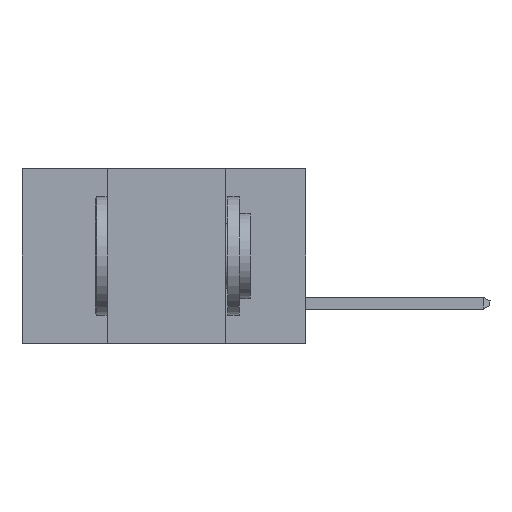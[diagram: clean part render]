
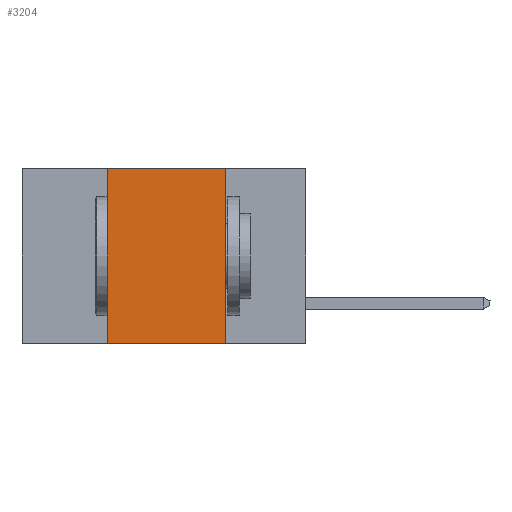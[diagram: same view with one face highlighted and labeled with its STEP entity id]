
A CAD part, left-side view. The second image highlights one B-rep face of the part: STEP entity #3204.
In plain terms, the highlighted planar face has unit normal (-1, 0, 0).
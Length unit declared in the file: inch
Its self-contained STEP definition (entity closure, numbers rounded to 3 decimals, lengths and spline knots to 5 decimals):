
#108 = VECTOR ( 'NONE', #5149, 39.37008 ) ;
#571 = CARTESIAN_POINT ( 'NONE',  ( 0., 0.42, 0. ) ) ;
#929 = LINE ( 'NONE', #991, #108 ) ;
#991 = CARTESIAN_POINT ( 'NONE',  ( 0., 0.6, 0. ) ) ;
#1037 = EDGE_CURVE ( 'NONE', #2066, #2470, #2763, .T. ) ;
#1097 = FACE_OUTER_BOUND ( 'NONE', #8620, .T. ) ;
#1545 = DIRECTION ( 'NONE',  ( 0., 0., -1. ) ) ;
#2066 = VERTEX_POINT ( 'NONE', #9506 ) ;
#2470 = VERTEX_POINT ( 'NONE', #571 ) ;
#2763 = LINE ( 'NONE', #6127, #11078 ) ;
#3100 = EDGE_CURVE ( 'NONE', #2066, #4912, #9475, .T. ) ;
#3168 = ORIENTED_EDGE ( 'NONE', *, *, #1037, .F. ) ;
#3204 = ADVANCED_FACE ( 'NONE', ( #1097 ), #3468, .F. ) ;
#3291 = CARTESIAN_POINT ( 'NONE',  ( 0., 0.17, -0.37 ) ) ;
#3309 = CARTESIAN_POINT ( 'NONE',  ( 0., 0.6, 0. ) ) ;
#3468 = PLANE ( 'NONE',  #12952 ) ;
#3511 = CARTESIAN_POINT ( 'NONE',  ( 0., 0.17, 0. ) ) ;
#4259 = DIRECTION ( 'NONE',  ( 0., -1., 0. ) ) ;
#4912 = VERTEX_POINT ( 'NONE', #3291 ) ;
#5149 = DIRECTION ( 'NONE',  ( 0., -1., 0. ) ) ;
#6127 = CARTESIAN_POINT ( 'NONE',  ( 0., 0.42, -0.37 ) ) ;
#6319 = CARTESIAN_POINT ( 'NONE',  ( 0., 0.6, -0.37 ) ) ;
#6654 = DIRECTION ( 'NONE',  ( 1., 0., 0. ) ) ;
#6657 = ORIENTED_EDGE ( 'NONE', *, *, #3100, .T. ) ;
#8009 = CARTESIAN_POINT ( 'NONE',  ( 0., 0.17, -0.37 ) ) ;
#8010 = VECTOR ( 'NONE', #1545, 39.37008 ) ;
#8293 = DIRECTION ( 'NONE',  ( 0., 0., 1. ) ) ;
#8620 = EDGE_LOOP ( 'NONE', ( #9438, #12912, #3168, #6657 ) ) ;
#8624 = DIRECTION ( 'NONE',  ( 0., 0., -1. ) ) ;
#9438 = ORIENTED_EDGE ( 'NONE', *, *, #12714, .F. ) ;
#9475 = LINE ( 'NONE', #6319, #10463 ) ;
#9506 = CARTESIAN_POINT ( 'NONE',  ( 0., 0.42, -0.37 ) ) ;
#10315 = LINE ( 'NONE', #8009, #8010 ) ;
#10463 = VECTOR ( 'NONE', #4259, 39.37008 ) ;
#10784 = VERTEX_POINT ( 'NONE', #3511 ) ;
#11078 = VECTOR ( 'NONE', #8293, 39.37008 ) ;
#12714 = EDGE_CURVE ( 'NONE', #10784, #4912, #10315, .T. ) ;
#12912 = ORIENTED_EDGE ( 'NONE', *, *, #13637, .F. ) ;
#12952 = AXIS2_PLACEMENT_3D ( 'NONE', #3309, #6654, #8624 ) ;
#13637 = EDGE_CURVE ( 'NONE', #2470, #10784, #929, .T. ) ;
